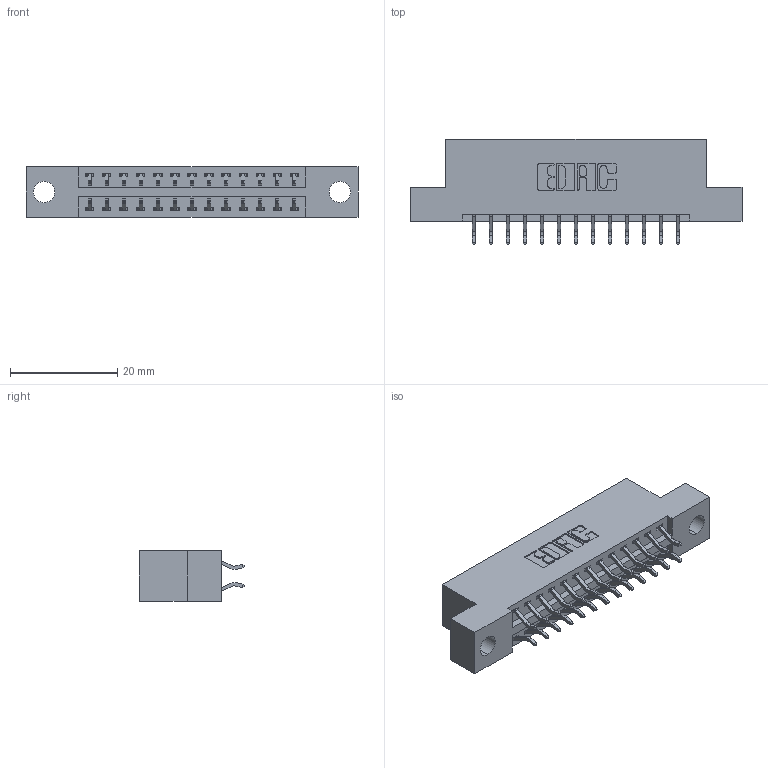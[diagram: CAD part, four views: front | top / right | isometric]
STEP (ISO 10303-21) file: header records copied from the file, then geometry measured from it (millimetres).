
FILE_DESCRIPTION (( 'STEP AP203' ), '1' );
FILE_NAME ('396-026-556-204.STEP', '2019-10-30T04:55:23', ( '' ), ( '' ), 'SwSTEP 2.0', 'SolidWorks 2016', '' );
FILE_SCHEMA (( 'CONFIG_CONTROL_DESIGN' ));
Length unit declared in the file: inch
Products named in the file (3): 345-292-001_556 Tail; 346 Part_Flush Mounting Lugs - 0.156 Dia-TH; 396-026-556-204
Assembly tree (27 placements, depth 2):
  396-026-556-204
    346 Part_Flush Mounting Lugs - 0.156 Dia-TH
    345-292-001_556 Tail  x26
Bounding box: 61.85 x 19.57 x 9.4 mm (x, y, z)
Volume: 5716.9 mm3; surface area: 7191.7 mm2
Topology: 27 solids, 27 shells, 1630 faces, 4827 edges, 3182 vertices
Faces by surface type: plane 1090, cylinder 540
Entity records: 12611 total; most frequent: CARTESIAN_POINT 2132, ORIENTED_EDGE 2054, DIRECTION 1919, EDGE_CURVE 1027, VECTOR 835, LINE 835, VERTEX_POINT 682, AXIS2_PLACEMENT_3D 542
